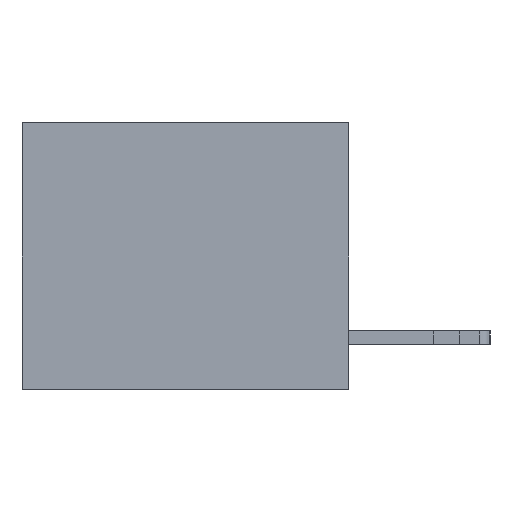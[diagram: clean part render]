
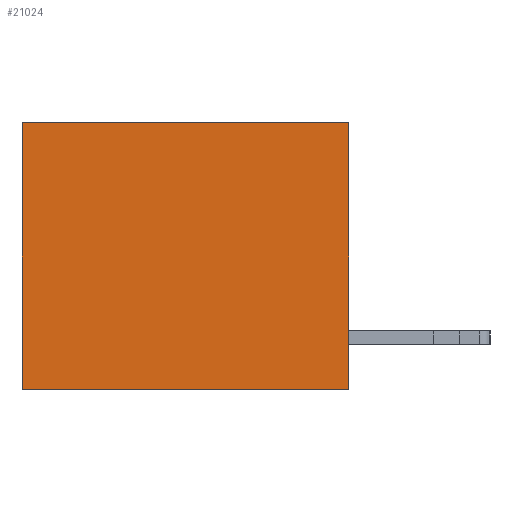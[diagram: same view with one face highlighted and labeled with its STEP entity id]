
A CAD part, left-side view. The second image highlights one B-rep face of the part: STEP entity #21024.
In plain terms, the highlighted planar face has unit normal (-1, 0, 0).
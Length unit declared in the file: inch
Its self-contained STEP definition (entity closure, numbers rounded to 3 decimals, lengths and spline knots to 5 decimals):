
#170 = CARTESIAN_POINT ( 'NONE',  ( 0.3165, 0., -0.49 ) ) ;
#208 = EDGE_LOOP ( 'NONE', ( #10125, #8705, #7907, #6888 ) ) ;
#513 = DIRECTION ( 'NONE',  ( 0., 1., 0. ) ) ;
#631 = CARTESIAN_POINT ( 'NONE',  ( 0.3165, 0., -0.49 ) ) ;
#1811 = LINE ( 'NONE', #15169, #10876 ) ;
#3112 = DIRECTION ( 'NONE',  ( 0., 1., 0. ) ) ;
#4834 = VERTEX_POINT ( 'NONE', #631 ) ;
#5334 = LINE ( 'NONE', #6157, #6871 ) ;
#6157 = CARTESIAN_POINT ( 'NONE',  ( 0.3165, 0.6, -0.49 ) ) ;
#6318 = CARTESIAN_POINT ( 'NONE',  ( 0.3165, 0., -0.49 ) ) ;
#6871 = VECTOR ( 'NONE', #14352, 39.37008 ) ;
#6888 = ORIENTED_EDGE ( 'NONE', *, *, #11344, .T. ) ;
#7320 = CARTESIAN_POINT ( 'NONE',  ( 0.3165, 0., 0. ) ) ;
#7907 = ORIENTED_EDGE ( 'NONE', *, *, #14443, .F. ) ;
#8387 = VECTOR ( 'NONE', #8732, 39.37008 ) ;
#8705 = ORIENTED_EDGE ( 'NONE', *, *, #14832, .F. ) ;
#8732 = DIRECTION ( 'NONE',  ( 0., 0., -1. ) ) ;
#9143 = LINE ( 'NONE', #6318, #15635 ) ;
#10125 = ORIENTED_EDGE ( 'NONE', *, *, #21266, .T. ) ;
#10876 = VECTOR ( 'NONE', #513, 39.37008 ) ;
#11344 = EDGE_CURVE ( 'NONE', #14178, #21280, #1811, .T. ) ;
#11664 = VERTEX_POINT ( 'NONE', #14279 ) ;
#12713 = AXIS2_PLACEMENT_3D ( 'NONE', #170, #13158, #13379 ) ;
#12804 = LINE ( 'NONE', #16793, #8387 ) ;
#13158 = DIRECTION ( 'NONE',  ( 1., 0., 0. ) ) ;
#13379 = DIRECTION ( 'NONE',  ( 0., 0., -1. ) ) ;
#14178 = VERTEX_POINT ( 'NONE', #7320 ) ;
#14279 = CARTESIAN_POINT ( 'NONE',  ( 0.3165, 0.6, -0.49 ) ) ;
#14352 = DIRECTION ( 'NONE',  ( 0., 0., -1. ) ) ;
#14443 = EDGE_CURVE ( 'NONE', #14178, #4834, #12804, .T. ) ;
#14832 = EDGE_CURVE ( 'NONE', #4834, #11664, #9143, .T. ) ;
#15169 = CARTESIAN_POINT ( 'NONE',  ( 0.3165, 0., 0. ) ) ;
#15635 = VECTOR ( 'NONE', #3112, 39.37008 ) ;
#16793 = CARTESIAN_POINT ( 'NONE',  ( 0.3165, 0., -0.49 ) ) ;
#17494 = CARTESIAN_POINT ( 'NONE',  ( 0.3165, 0.6, 0. ) ) ;
#19086 = FACE_OUTER_BOUND ( 'NONE', #208, .T. ) ;
#19682 = PLANE ( 'NONE',  #12713 ) ;
#21024 = ADVANCED_FACE ( 'NONE', ( #19086 ), #19682, .F. ) ;
#21266 = EDGE_CURVE ( 'NONE', #21280, #11664, #5334, .T. ) ;
#21280 = VERTEX_POINT ( 'NONE', #17494 ) ;
